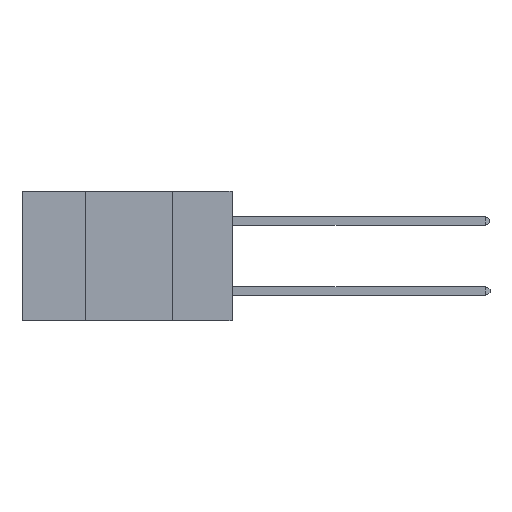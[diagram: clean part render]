
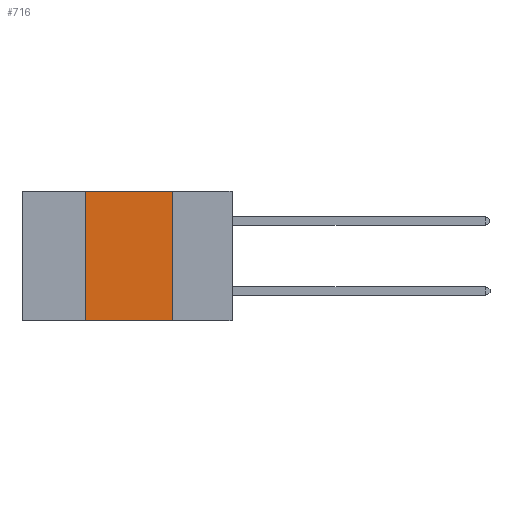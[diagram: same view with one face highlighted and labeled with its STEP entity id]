
A CAD part, left-side view. The second image highlights one B-rep face of the part: STEP entity #716.
In plain terms, the highlighted planar face has unit normal (-1, 0, 0).
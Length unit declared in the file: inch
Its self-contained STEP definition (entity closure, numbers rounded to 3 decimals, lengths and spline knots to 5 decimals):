
#72 = DIRECTION ( 'NONE',  ( 1., 0., 0. ) ) ;
#164 = CARTESIAN_POINT ( 'NONE',  ( 0., 0.17, -0.37 ) ) ;
#241 = DIRECTION ( 'NONE',  ( 0., 0., -1. ) ) ;
#632 = CARTESIAN_POINT ( 'NONE',  ( 0., 0.6, -0.37 ) ) ;
#716 = ADVANCED_FACE ( 'NONE', ( #6654 ), #985, .F. ) ;
#834 = CARTESIAN_POINT ( 'NONE',  ( 0., 0.42, 0. ) ) ;
#985 = PLANE ( 'NONE',  #7405 ) ;
#1197 = ORIENTED_EDGE ( 'NONE', *, *, #9305, .T. ) ;
#1215 = CARTESIAN_POINT ( 'NONE',  ( 0., 0.6, 0. ) ) ;
#1404 = VERTEX_POINT ( 'NONE', #834 ) ;
#2021 = VECTOR ( 'NONE', #3411, 39.37008 ) ;
#2363 = LINE ( 'NONE', #4757, #2021 ) ;
#2393 = VECTOR ( 'NONE', #4573, 39.37008 ) ;
#2423 = EDGE_CURVE ( 'NONE', #6610, #1404, #2363, .T. ) ;
#3411 = DIRECTION ( 'NONE',  ( 0., 0., 1. ) ) ;
#4034 = ORIENTED_EDGE ( 'NONE', *, *, #2423, .F. ) ;
#4573 = DIRECTION ( 'NONE',  ( 0., 0., -1. ) ) ;
#4757 = CARTESIAN_POINT ( 'NONE',  ( 0., 0.42, 0. ) ) ;
#5503 = ORIENTED_EDGE ( 'NONE', *, *, #9522, .F. ) ;
#6126 = EDGE_LOOP ( 'NONE', ( #7816, #5503, #4034, #1197 ) ) ;
#6169 = VECTOR ( 'NONE', #9095, 39.37008 ) ;
#6336 = LINE ( 'NONE', #632, #8874 ) ;
#6347 = VERTEX_POINT ( 'NONE', #164 ) ;
#6610 = VERTEX_POINT ( 'NONE', #7800 ) ;
#6654 = FACE_OUTER_BOUND ( 'NONE', #6126, .T. ) ;
#7280 = CARTESIAN_POINT ( 'NONE',  ( 0., 0.17, 0. ) ) ;
#7405 = AXIS2_PLACEMENT_3D ( 'NONE', #1215, #72, #241 ) ;
#7602 = CARTESIAN_POINT ( 'NONE',  ( 0., 0.17, 0. ) ) ;
#7800 = CARTESIAN_POINT ( 'NONE',  ( 0., 0.42, -0.37 ) ) ;
#7816 = ORIENTED_EDGE ( 'NONE', *, *, #7955, .F. ) ;
#7955 = EDGE_CURVE ( 'NONE', #12669, #6347, #12076, .T. ) ;
#8729 = LINE ( 'NONE', #11788, #6169 ) ;
#8874 = VECTOR ( 'NONE', #11509, 39.37008 ) ;
#9095 = DIRECTION ( 'NONE',  ( 0., -1., 0. ) ) ;
#9305 = EDGE_CURVE ( 'NONE', #6610, #6347, #6336, .T. ) ;
#9522 = EDGE_CURVE ( 'NONE', #1404, #12669, #8729, .T. ) ;
#11509 = DIRECTION ( 'NONE',  ( 0., -1., 0. ) ) ;
#11788 = CARTESIAN_POINT ( 'NONE',  ( 0., 0.6, 0. ) ) ;
#12076 = LINE ( 'NONE', #7602, #2393 ) ;
#12669 = VERTEX_POINT ( 'NONE', #7280 ) ;
